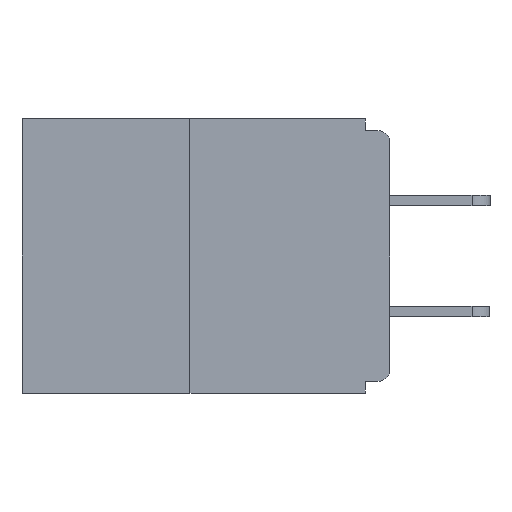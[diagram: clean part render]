
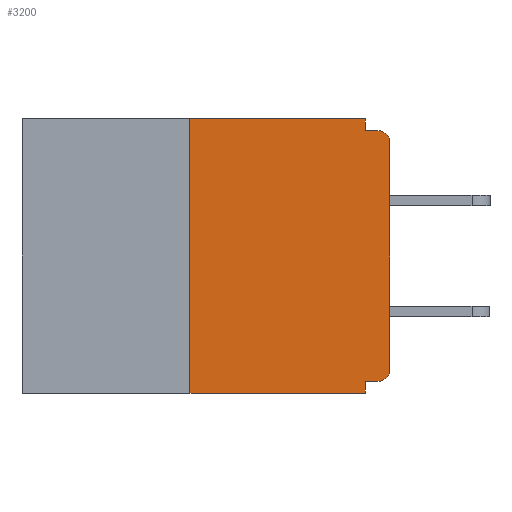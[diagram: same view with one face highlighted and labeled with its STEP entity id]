
A CAD part, left-side view. The second image highlights one B-rep face of the part: STEP entity #3200.
In plain terms, the highlighted planar face has unit normal (-1, 0, 0).
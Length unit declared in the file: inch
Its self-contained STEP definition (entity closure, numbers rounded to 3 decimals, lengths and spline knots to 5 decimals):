
#485 = VECTOR ( 'NONE', #7194, 39.37008 ) ;
#788 = LINE ( 'NONE', #15753, #12290 ) ;
#951 = PLANE ( 'NONE',  #15056 ) ;
#1157 = DIRECTION ( 'NONE',  ( 0., 0., 1. ) ) ;
#1167 = DIRECTION ( 'NONE',  ( 0., 0., -1. ) ) ;
#1220 = CARTESIAN_POINT ( 'NONE',  ( 0., 0., -0.03 ) ) ;
#1361 = EDGE_CURVE ( 'NONE', #14400, #16020, #12046, .T. ) ;
#1421 = EDGE_CURVE ( 'NONE', #17801, #12315, #7085, .T. ) ;
#1540 = LINE ( 'NONE', #13833, #485 ) ;
#1719 = CIRCLE ( 'NONE', #12369, 0.015 ) ;
#2049 = ORIENTED_EDGE ( 'NONE', *, *, #1361, .T. ) ;
#2260 = CARTESIAN_POINT ( 'NONE',  ( 0., 0.25, 0. ) ) ;
#3200 = ADVANCED_FACE ( 'NONE', ( #3617 ), #951, .F. ) ;
#3308 = LINE ( 'NONE', #15727, #9029 ) ;
#3419 = VECTOR ( 'NONE', #17621, 39.37008 ) ;
#3617 = FACE_OUTER_BOUND ( 'NONE', #16774, .T. ) ;
#3652 = ORIENTED_EDGE ( 'NONE', *, *, #1421, .F. ) ;
#3875 = LINE ( 'NONE', #8661, #5937 ) ;
#4242 = DIRECTION ( 'NONE',  ( 0., 0., -1. ) ) ;
#4316 = DIRECTION ( 'NONE',  ( 1., 0., 0. ) ) ;
#4380 = CARTESIAN_POINT ( 'NONE',  ( 0., 0.015, -0.03 ) ) ;
#4419 = ORIENTED_EDGE ( 'NONE', *, *, #10271, .T. ) ;
#4521 = EDGE_CURVE ( 'NONE', #12904, #11915, #5066, .T. ) ;
#4574 = CARTESIAN_POINT ( 'NONE',  ( 0., 0., 0. ) ) ;
#4614 = AXIS2_PLACEMENT_3D ( 'NONE', #16481, #19893, #4943 ) ;
#4943 = DIRECTION ( 'NONE',  ( 0., 0., -1. ) ) ;
#5066 = LINE ( 'NONE', #2260, #12890 ) ;
#5489 = LINE ( 'NONE', #12314, #3419 ) ;
#5773 = VERTEX_POINT ( 'NONE', #20064 ) ;
#5937 = VECTOR ( 'NONE', #18652, 39.37008 ) ;
#5985 = ORIENTED_EDGE ( 'NONE', *, *, #6270, .F. ) ;
#6040 = DIRECTION ( 'NONE',  ( -1., 0., 0. ) ) ;
#6270 = EDGE_CURVE ( 'NONE', #11915, #5773, #5489, .T. ) ;
#6630 = CARTESIAN_POINT ( 'NONE',  ( 0., 0.015, -0.328 ) ) ;
#6961 = EDGE_CURVE ( 'NONE', #14400, #13101, #1540, .T. ) ;
#7085 = LINE ( 'NONE', #21164, #15492 ) ;
#7111 = VERTEX_POINT ( 'NONE', #13441 ) ;
#7194 = DIRECTION ( 'NONE',  ( 0., 1., 0. ) ) ;
#7523 = DIRECTION ( 'NONE',  ( 0., -1., 0. ) ) ;
#7556 = DIRECTION ( 'NONE',  ( 0., -1., 0. ) ) ;
#8429 = ORIENTED_EDGE ( 'NONE', *, *, #15291, .F. ) ;
#8661 = CARTESIAN_POINT ( 'NONE',  ( 0., 0.031, 0. ) ) ;
#9029 = VECTOR ( 'NONE', #7556, 39.37008 ) ;
#9253 = ORIENTED_EDGE ( 'NONE', *, *, #6961, .F. ) ;
#9729 = CARTESIAN_POINT ( 'NONE',  ( 0., 0.031, -0.328 ) ) ;
#10271 = EDGE_CURVE ( 'NONE', #16020, #19416, #20067, .T. ) ;
#10932 = CARTESIAN_POINT ( 'NONE',  ( 0., 0.25, 0. ) ) ;
#11837 = ORIENTED_EDGE ( 'NONE', *, *, #19290, .F. ) ;
#11915 = VERTEX_POINT ( 'NONE', #10932 ) ;
#12046 = CIRCLE ( 'NONE', #4614, 0.015 ) ;
#12290 = VECTOR ( 'NONE', #14138, 39.37008 ) ;
#12314 = CARTESIAN_POINT ( 'NONE',  ( 0., 0.46, 0. ) ) ;
#12315 = VERTEX_POINT ( 'NONE', #12608 ) ;
#12352 = CARTESIAN_POINT ( 'NONE',  ( 0., 0.031, -0.015 ) ) ;
#12369 = AXIS2_PLACEMENT_3D ( 'NONE', #4380, #6040, #1167 ) ;
#12608 = CARTESIAN_POINT ( 'NONE',  ( 0., 0.015, -0.015 ) ) ;
#12890 = VECTOR ( 'NONE', #13868, 39.37008 ) ;
#12904 = VERTEX_POINT ( 'NONE', #21250 ) ;
#13101 = VERTEX_POINT ( 'NONE', #9729 ) ;
#13441 = CARTESIAN_POINT ( 'NONE',  ( 0., 0.031, -0.343 ) ) ;
#13833 = CARTESIAN_POINT ( 'NONE',  ( 0., 0., -0.328 ) ) ;
#13868 = DIRECTION ( 'NONE',  ( 0., 0., 1. ) ) ;
#14025 = ORIENTED_EDGE ( 'NONE', *, *, #4521, .F. ) ;
#14138 = DIRECTION ( 'NONE',  ( 0., 0., -1. ) ) ;
#14400 = VERTEX_POINT ( 'NONE', #6630 ) ;
#15022 = ORIENTED_EDGE ( 'NONE', *, *, #15964, .T. ) ;
#15056 = AXIS2_PLACEMENT_3D ( 'NONE', #21099, #4316, #4242 ) ;
#15291 = EDGE_CURVE ( 'NONE', #5773, #17801, #3875, .T. ) ;
#15492 = VECTOR ( 'NONE', #7523, 39.37008 ) ;
#15727 = CARTESIAN_POINT ( 'NONE',  ( 0., 0.46, -0.343 ) ) ;
#15753 = CARTESIAN_POINT ( 'NONE',  ( 0., 0.031, -0.343 ) ) ;
#15964 = EDGE_CURVE ( 'NONE', #12904, #7111, #3308, .T. ) ;
#16020 = VERTEX_POINT ( 'NONE', #19686 ) ;
#16250 = EDGE_CURVE ( 'NONE', #19416, #12315, #1719, .T. ) ;
#16481 = CARTESIAN_POINT ( 'NONE',  ( 0., 0.015, -0.313 ) ) ;
#16614 = VECTOR ( 'NONE', #1157, 39.37008 ) ;
#16774 = EDGE_LOOP ( 'NONE', ( #5985, #14025, #15022, #11837, #9253, #2049, #4419, #20288, #3652, #8429 ) ) ;
#17621 = DIRECTION ( 'NONE',  ( 0., -1., 0. ) ) ;
#17801 = VERTEX_POINT ( 'NONE', #12352 ) ;
#18652 = DIRECTION ( 'NONE',  ( 0., 0., -1. ) ) ;
#19290 = EDGE_CURVE ( 'NONE', #13101, #7111, #788, .T. ) ;
#19416 = VERTEX_POINT ( 'NONE', #1220 ) ;
#19686 = CARTESIAN_POINT ( 'NONE',  ( 0., 0., -0.313 ) ) ;
#19893 = DIRECTION ( 'NONE',  ( -1., 0., 0. ) ) ;
#20064 = CARTESIAN_POINT ( 'NONE',  ( 0., 0.031, 0. ) ) ;
#20067 = LINE ( 'NONE', #4574, #16614 ) ;
#20288 = ORIENTED_EDGE ( 'NONE', *, *, #16250, .T. ) ;
#21099 = CARTESIAN_POINT ( 'NONE',  ( 0., 0.46, 0. ) ) ;
#21164 = CARTESIAN_POINT ( 'NONE',  ( 0., 0., -0.015 ) ) ;
#21250 = CARTESIAN_POINT ( 'NONE',  ( 0., 0.25, -0.343 ) ) ;
